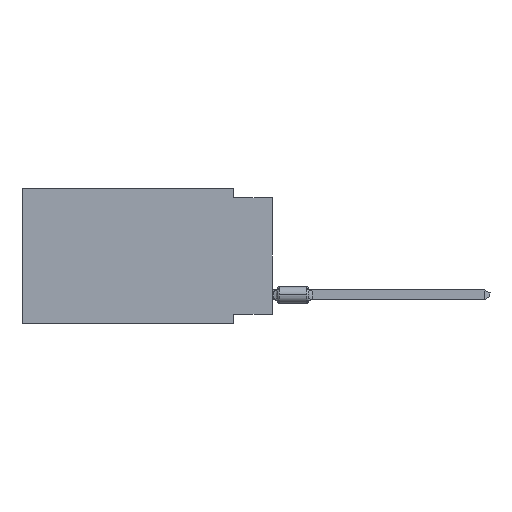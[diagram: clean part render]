
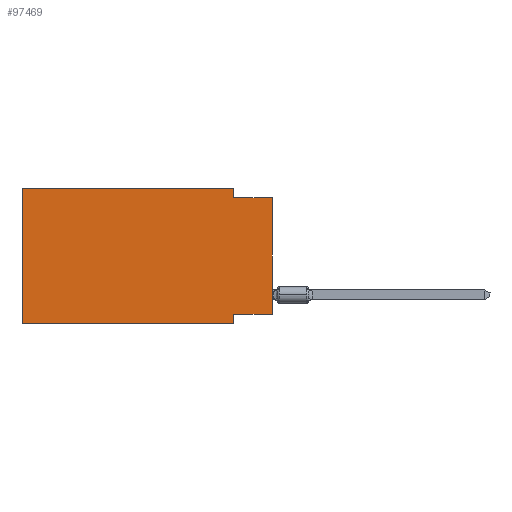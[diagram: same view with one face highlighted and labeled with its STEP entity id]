
A CAD part, left-side view. The second image highlights one B-rep face of the part: STEP entity #97469.
In plain terms, the highlighted planar face has unit normal (-1, 0, 0).
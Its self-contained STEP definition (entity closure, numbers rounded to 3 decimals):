
#2303 = LINE ( 'NONE', #59212, #89443 ) ;
#5462 = VECTOR ( 'NONE', #45557, 1000. ) ;
#7030 = DIRECTION ( 'NONE',  ( 1., 0., 0. ) ) ;
#7301 = DIRECTION ( 'NONE',  ( 0., 0., -1. ) ) ;
#8099 = CARTESIAN_POINT ( 'NONE',  ( 0., 16.383, 0. ) ) ;
#12884 = DIRECTION ( 'NONE',  ( 0., 0., 1. ) ) ;
#14463 = LINE ( 'NONE', #99207, #94338 ) ;
#16152 = ORIENTED_EDGE ( 'NONE', *, *, #94456, .F. ) ;
#16790 = CARTESIAN_POINT ( 'NONE',  ( 0., 0., 0. ) ) ;
#19591 = LINE ( 'NONE', #53634, #86955 ) ;
#22242 = CARTESIAN_POINT ( 'NONE',  ( 0., 16.383, 0. ) ) ;
#23023 = ORIENTED_EDGE ( 'NONE', *, *, #46608, .F. ) ;
#23515 = CARTESIAN_POINT ( 'NONE',  ( 0., 2.54, -8.255 ) ) ;
#23581 = VERTEX_POINT ( 'NONE', #33597 ) ;
#23696 = VERTEX_POINT ( 'NONE', #54178 ) ;
#27657 = ORIENTED_EDGE ( 'NONE', *, *, #76428, .T. ) ;
#28245 = CARTESIAN_POINT ( 'NONE',  ( 0., 2.54, -8.89 ) ) ;
#28601 = VECTOR ( 'NONE', #47758, 1000. ) ;
#30313 = CARTESIAN_POINT ( 'NONE',  ( 0., 0., -0.635 ) ) ;
#31734 = DIRECTION ( 'NONE',  ( 0., -1., 0. ) ) ;
#33597 = CARTESIAN_POINT ( 'NONE',  ( 0., 16.383, -8.89 ) ) ;
#41194 = DIRECTION ( 'NONE',  ( 0., -1., 0. ) ) ;
#41777 = EDGE_CURVE ( 'NONE', #93101, #70167, #69178, .T. ) ;
#44276 = CARTESIAN_POINT ( 'NONE',  ( 0., 2.54, 0. ) ) ;
#45557 = DIRECTION ( 'NONE',  ( 0., 0., -1. ) ) ;
#46608 = EDGE_CURVE ( 'NONE', #87806, #81985, #84114, .T. ) ;
#47758 = DIRECTION ( 'NONE',  ( 0., 1., 0. ) ) ;
#49404 = PLANE ( 'NONE',  #84655 ) ;
#51044 = FACE_OUTER_BOUND ( 'NONE', #105757, .T. ) ;
#51241 = CARTESIAN_POINT ( 'NONE',  ( 0., 0., -8.255 ) ) ;
#51677 = CARTESIAN_POINT ( 'NONE',  ( 0., 16.383, 0. ) ) ;
#51919 = DIRECTION ( 'NONE',  ( 0., 0., 1. ) ) ;
#52384 = CARTESIAN_POINT ( 'NONE',  ( 0., 2.54, -0.635 ) ) ;
#53178 = EDGE_CURVE ( 'NONE', #87478, #23696, #105736, .T. ) ;
#53634 = CARTESIAN_POINT ( 'NONE',  ( 0., 16.383, 0. ) ) ;
#54178 = CARTESIAN_POINT ( 'NONE',  ( 0., 2.54, -8.89 ) ) ;
#58038 = CARTESIAN_POINT ( 'NONE',  ( 0., 2.54, 0. ) ) ;
#59212 = CARTESIAN_POINT ( 'NONE',  ( 0., 0., -0.635 ) ) ;
#60352 = VECTOR ( 'NONE', #51919, 1000. ) ;
#60548 = ORIENTED_EDGE ( 'NONE', *, *, #100395, .F. ) ;
#68659 = ORIENTED_EDGE ( 'NONE', *, *, #41777, .T. ) ;
#68759 = VERTEX_POINT ( 'NONE', #52384 ) ;
#69178 = LINE ( 'NONE', #16790, #60352 ) ;
#70167 = VERTEX_POINT ( 'NONE', #30313 ) ;
#70714 = EDGE_CURVE ( 'NONE', #81985, #68759, #84218, .T. ) ;
#75324 = ORIENTED_EDGE ( 'NONE', *, *, #70714, .F. ) ;
#76428 = EDGE_CURVE ( 'NONE', #23581, #23696, #14463, .T. ) ;
#81985 = VERTEX_POINT ( 'NONE', #44276 ) ;
#83915 = ORIENTED_EDGE ( 'NONE', *, *, #92095, .F. ) ;
#84114 = LINE ( 'NONE', #22242, #97128 ) ;
#84218 = LINE ( 'NONE', #58038, #98514 ) ;
#84655 = AXIS2_PLACEMENT_3D ( 'NONE', #8099, #7030, #100116 ) ;
#86955 = VECTOR ( 'NONE', #12884, 1000. ) ;
#87478 = VERTEX_POINT ( 'NONE', #23515 ) ;
#87806 = VERTEX_POINT ( 'NONE', #51677 ) ;
#89443 = VECTOR ( 'NONE', #93209, 1000. ) ;
#91222 = LINE ( 'NONE', #106836, #28601 ) ;
#92095 = EDGE_CURVE ( 'NONE', #93101, #87478, #91222, .T. ) ;
#93101 = VERTEX_POINT ( 'NONE', #51241 ) ;
#93209 = DIRECTION ( 'NONE',  ( 0., -1., 0. ) ) ;
#94338 = VECTOR ( 'NONE', #31734, 1000. ) ;
#94456 = EDGE_CURVE ( 'NONE', #68759, #70167, #2303, .T. ) ;
#97128 = VECTOR ( 'NONE', #41194, 1000. ) ;
#97469 = ADVANCED_FACE ( 'NONE', ( #51044 ), #49404, .F. ) ;
#98514 = VECTOR ( 'NONE', #7301, 1000. ) ;
#99207 = CARTESIAN_POINT ( 'NONE',  ( 0., 16.383, -8.89 ) ) ;
#100116 = DIRECTION ( 'NONE',  ( 0., 0., -1. ) ) ;
#100395 = EDGE_CURVE ( 'NONE', #23581, #87806, #19591, .T. ) ;
#105736 = LINE ( 'NONE', #28245, #5462 ) ;
#105757 = EDGE_LOOP ( 'NONE', ( #68659, #16152, #75324, #23023, #60548, #27657, #110097, #83915 ) ) ;
#106836 = CARTESIAN_POINT ( 'NONE',  ( 0., 0., -8.255 ) ) ;
#110097 = ORIENTED_EDGE ( 'NONE', *, *, #53178, .F. ) ;
